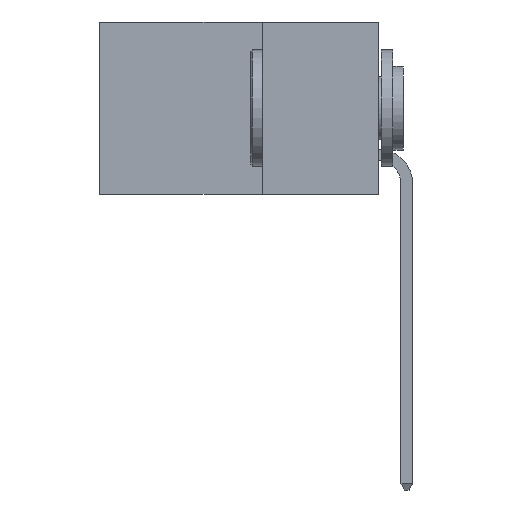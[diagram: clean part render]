
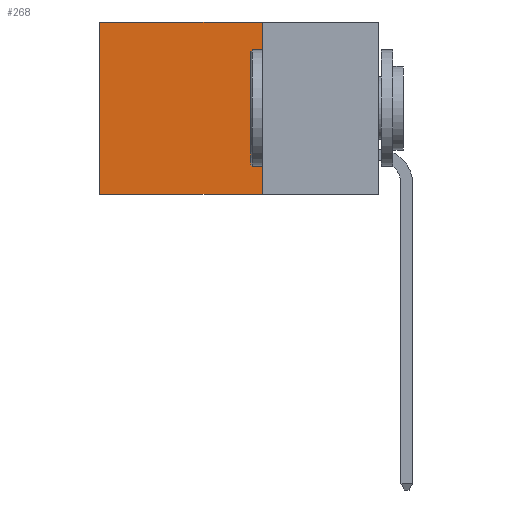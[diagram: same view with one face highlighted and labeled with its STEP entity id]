
A CAD part, left-side view. The second image highlights one B-rep face of the part: STEP entity #268.
In plain terms, the highlighted planar face has unit normal (-1, 0, 0).
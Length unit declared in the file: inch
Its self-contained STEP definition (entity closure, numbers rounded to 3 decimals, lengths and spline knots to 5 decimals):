
#268 = ADVANCED_FACE ( 'NONE', ( #3702 ), #10668, .F. ) ;
#1788 = CARTESIAN_POINT ( 'NONE',  ( 0.2615, 0.6, -0.37 ) ) ;
#1795 = LINE ( 'NONE', #4328, #3814 ) ;
#1877 = DIRECTION ( 'NONE',  ( 1., 0., 0. ) ) ;
#2940 = EDGE_LOOP ( 'NONE', ( #11001, #10768, #3462, #8583 ) ) ;
#3020 = VECTOR ( 'NONE', #9474, 39.37008 ) ;
#3368 = VERTEX_POINT ( 'NONE', #8465 ) ;
#3462 = ORIENTED_EDGE ( 'NONE', *, *, #8961, .F. ) ;
#3702 = FACE_OUTER_BOUND ( 'NONE', #2940, .T. ) ;
#3814 = VECTOR ( 'NONE', #6106, 39.37008 ) ;
#4265 = VERTEX_POINT ( 'NONE', #1788 ) ;
#4328 = CARTESIAN_POINT ( 'NONE',  ( 0.2615, 0.25, -0.37 ) ) ;
#4557 = AXIS2_PLACEMENT_3D ( 'NONE', #6171, #1877, #4621 ) ;
#4621 = DIRECTION ( 'NONE',  ( 0., 0., -1. ) ) ;
#5013 = CARTESIAN_POINT ( 'NONE',  ( 0.2615, 0.6, 0. ) ) ;
#5330 = LINE ( 'NONE', #10485, #9552 ) ;
#6106 = DIRECTION ( 'NONE',  ( 0., 1., 0. ) ) ;
#6171 = CARTESIAN_POINT ( 'NONE',  ( 0.2615, 0.25, -0.37 ) ) ;
#6329 = CARTESIAN_POINT ( 'NONE',  ( 0.2615, 0.25, -0.37 ) ) ;
#6701 = LINE ( 'NONE', #9229, #8645 ) ;
#7386 = EDGE_CURVE ( 'NONE', #10128, #4265, #9801, .T. ) ;
#7483 = VERTEX_POINT ( 'NONE', #6329 ) ;
#7636 = DIRECTION ( 'NONE',  ( 0., 0., -1. ) ) ;
#8465 = CARTESIAN_POINT ( 'NONE',  ( 0.2615, 0.25, 0. ) ) ;
#8553 = EDGE_CURVE ( 'NONE', #7483, #4265, #1795, .T. ) ;
#8583 = ORIENTED_EDGE ( 'NONE', *, *, #10981, .T. ) ;
#8645 = VECTOR ( 'NONE', #7636, 39.37008 ) ;
#8941 = DIRECTION ( 'NONE',  ( 0., 1., 0. ) ) ;
#8961 = EDGE_CURVE ( 'NONE', #3368, #7483, #6701, .T. ) ;
#9229 = CARTESIAN_POINT ( 'NONE',  ( 0.2615, 0.25, -0.37 ) ) ;
#9474 = DIRECTION ( 'NONE',  ( 0., 0., -1. ) ) ;
#9552 = VECTOR ( 'NONE', #8941, 39.37008 ) ;
#9801 = LINE ( 'NONE', #10288, #3020 ) ;
#10128 = VERTEX_POINT ( 'NONE', #5013 ) ;
#10288 = CARTESIAN_POINT ( 'NONE',  ( 0.2615, 0.6, -0.37 ) ) ;
#10485 = CARTESIAN_POINT ( 'NONE',  ( 0.2615, 0.25, 0. ) ) ;
#10668 = PLANE ( 'NONE',  #4557 ) ;
#10768 = ORIENTED_EDGE ( 'NONE', *, *, #8553, .F. ) ;
#10981 = EDGE_CURVE ( 'NONE', #3368, #10128, #5330, .T. ) ;
#11001 = ORIENTED_EDGE ( 'NONE', *, *, #7386, .T. ) ;
